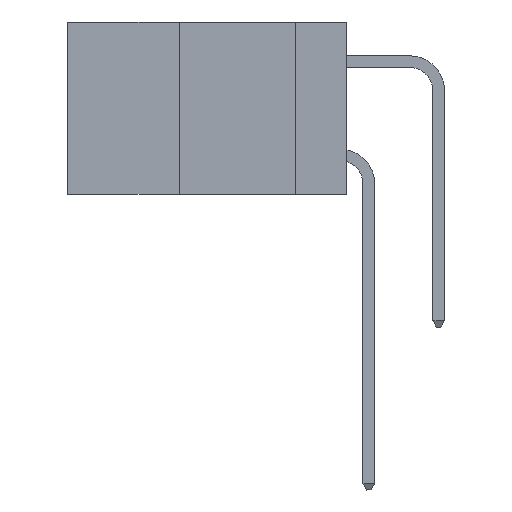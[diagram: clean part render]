
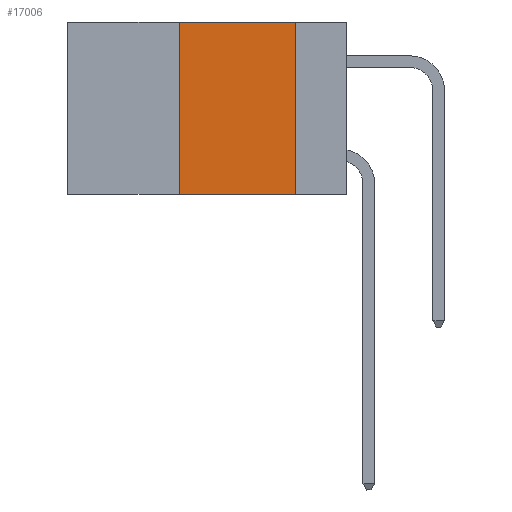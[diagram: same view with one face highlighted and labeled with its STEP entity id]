
A CAD part, left-side view. The second image highlights one B-rep face of the part: STEP entity #17006.
In plain terms, the highlighted planar face has unit normal (-1, 0, 0).
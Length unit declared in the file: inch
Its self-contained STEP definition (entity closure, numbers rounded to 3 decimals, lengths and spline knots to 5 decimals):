
#56 = CARTESIAN_POINT ( 'NONE',  ( 0., 0.36, 0. ) ) ;
#1245 = DIRECTION ( 'NONE',  ( 1., 0., 0. ) ) ;
#1267 = CARTESIAN_POINT ( 'NONE',  ( 0., 0.36, 0. ) ) ;
#1344 = EDGE_LOOP ( 'NONE', ( #10882, #6877, #1538, #17815 ) ) ;
#1538 = ORIENTED_EDGE ( 'NONE', *, *, #16500, .F. ) ;
#2624 = VERTEX_POINT ( 'NONE', #8604 ) ;
#2632 = DIRECTION ( 'NONE',  ( 0., 0., 1. ) ) ;
#2937 = VECTOR ( 'NONE', #18548, 39.37008 ) ;
#3231 = VECTOR ( 'NONE', #17586, 39.37008 ) ;
#3424 = VERTEX_POINT ( 'NONE', #6490 ) ;
#4701 = AXIS2_PLACEMENT_3D ( 'NONE', #13755, #1245, #20093 ) ;
#4882 = FACE_OUTER_BOUND ( 'NONE', #1344, .T. ) ;
#5389 = LINE ( 'NONE', #11649, #19848 ) ;
#6052 = DIRECTION ( 'NONE',  ( 0., 0., -1. ) ) ;
#6490 = CARTESIAN_POINT ( 'NONE',  ( 0., 0.11, -0.37 ) ) ;
#6677 = LINE ( 'NONE', #6739, #3231 ) ;
#6739 = CARTESIAN_POINT ( 'NONE',  ( 0., 0.6, -0.37 ) ) ;
#6877 = ORIENTED_EDGE ( 'NONE', *, *, #11727, .F. ) ;
#8604 = CARTESIAN_POINT ( 'NONE',  ( 0., 0.36, -0.37 ) ) ;
#9078 = LINE ( 'NONE', #20107, #2937 ) ;
#10823 = EDGE_CURVE ( 'NONE', #2624, #3424, #6677, .T. ) ;
#10882 = ORIENTED_EDGE ( 'NONE', *, *, #15782, .F. ) ;
#11447 = LINE ( 'NONE', #1267, #18379 ) ;
#11649 = CARTESIAN_POINT ( 'NONE',  ( 0., 0.11, 0. ) ) ;
#11727 = EDGE_CURVE ( 'NONE', #14809, #15550, #9078, .T. ) ;
#13755 = CARTESIAN_POINT ( 'NONE',  ( 0., 0.6, 0. ) ) ;
#14809 = VERTEX_POINT ( 'NONE', #56 ) ;
#15530 = PLANE ( 'NONE',  #4701 ) ;
#15550 = VERTEX_POINT ( 'NONE', #18340 ) ;
#15782 = EDGE_CURVE ( 'NONE', #15550, #3424, #5389, .T. ) ;
#16500 = EDGE_CURVE ( 'NONE', #2624, #14809, #11447, .T. ) ;
#17006 = ADVANCED_FACE ( 'NONE', ( #4882 ), #15530, .F. ) ;
#17586 = DIRECTION ( 'NONE',  ( 0., -1., 0. ) ) ;
#17815 = ORIENTED_EDGE ( 'NONE', *, *, #10823, .T. ) ;
#18340 = CARTESIAN_POINT ( 'NONE',  ( 0., 0.11, 0. ) ) ;
#18379 = VECTOR ( 'NONE', #2632, 39.37008 ) ;
#18548 = DIRECTION ( 'NONE',  ( 0., -1., 0. ) ) ;
#19848 = VECTOR ( 'NONE', #6052, 39.37008 ) ;
#20093 = DIRECTION ( 'NONE',  ( 0., 0., -1. ) ) ;
#20107 = CARTESIAN_POINT ( 'NONE',  ( 0., 0.6, 0. ) ) ;
